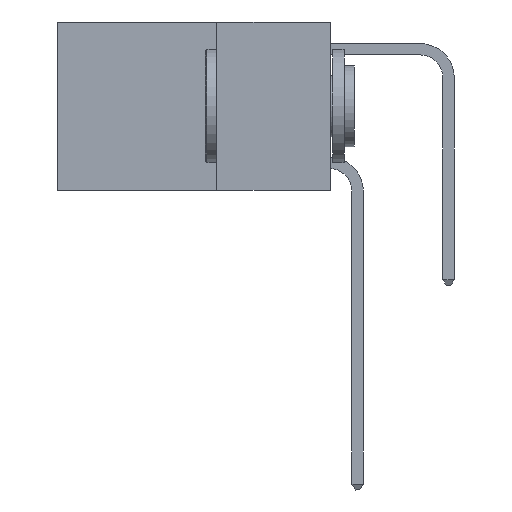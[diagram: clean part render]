
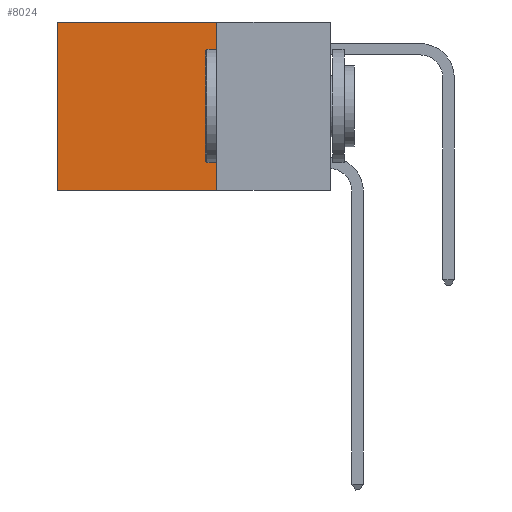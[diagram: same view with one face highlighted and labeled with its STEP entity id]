
A CAD part, left-side view. The second image highlights one B-rep face of the part: STEP entity #8024.
In plain terms, the highlighted planar face has unit normal (-1, 0, 0).
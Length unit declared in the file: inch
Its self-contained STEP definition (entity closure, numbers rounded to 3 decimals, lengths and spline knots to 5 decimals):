
#438 = DIRECTION ( 'NONE',  ( 0., 1., 0. ) ) ;
#1142 = VECTOR ( 'NONE', #12950, 39.37008 ) ;
#1522 = ORIENTED_EDGE ( 'NONE', *, *, #3613, .T. ) ;
#1818 = ORIENTED_EDGE ( 'NONE', *, *, #5618, .F. ) ;
#2028 = CARTESIAN_POINT ( 'NONE',  ( 0.2625, 0.6, 0. ) ) ;
#2216 = CARTESIAN_POINT ( 'NONE',  ( 0.2625, 0.25, 0. ) ) ;
#2420 = LINE ( 'NONE', #7058, #2683 ) ;
#2637 = VECTOR ( 'NONE', #438, 39.37008 ) ;
#2656 = CARTESIAN_POINT ( 'NONE',  ( 0.2625, 0.25, 0. ) ) ;
#2683 = VECTOR ( 'NONE', #15182, 39.37008 ) ;
#2760 = CARTESIAN_POINT ( 'NONE',  ( 0.2625, 0.6, 0. ) ) ;
#2827 = LINE ( 'NONE', #2760, #7575 ) ;
#3084 = VERTEX_POINT ( 'NONE', #2028 ) ;
#3613 = EDGE_CURVE ( 'NONE', #12579, #3084, #4598, .T. ) ;
#3783 = EDGE_CURVE ( 'NONE', #5805, #8089, #14579, .T. ) ;
#3784 = EDGE_CURVE ( 'NONE', #3084, #8089, #2827, .T. ) ;
#4338 = EDGE_LOOP ( 'NONE', ( #11737, #5523, #1818, #1522 ) ) ;
#4598 = LINE ( 'NONE', #2216, #1142 ) ;
#4959 = AXIS2_PLACEMENT_3D ( 'NONE', #7423, #13284, #6331 ) ;
#5523 = ORIENTED_EDGE ( 'NONE', *, *, #3783, .F. ) ;
#5618 = EDGE_CURVE ( 'NONE', #12579, #5805, #2420, .T. ) ;
#5805 = VERTEX_POINT ( 'NONE', #8611 ) ;
#6193 = FACE_OUTER_BOUND ( 'NONE', #4338, .T. ) ;
#6331 = DIRECTION ( 'NONE',  ( 0., 0., -1. ) ) ;
#7058 = CARTESIAN_POINT ( 'NONE',  ( 0.2625, 0.25, 0. ) ) ;
#7423 = CARTESIAN_POINT ( 'NONE',  ( 0.2625, 0.25, 0. ) ) ;
#7575 = VECTOR ( 'NONE', #11085, 39.37008 ) ;
#8024 = ADVANCED_FACE ( 'NONE', ( #6193 ), #8575, .F. ) ;
#8089 = VERTEX_POINT ( 'NONE', #9236 ) ;
#8575 = PLANE ( 'NONE',  #4959 ) ;
#8611 = CARTESIAN_POINT ( 'NONE',  ( 0.2625, 0.25, -0.37 ) ) ;
#9236 = CARTESIAN_POINT ( 'NONE',  ( 0.2625, 0.6, -0.37 ) ) ;
#10937 = CARTESIAN_POINT ( 'NONE',  ( 0.2625, 0.25, -0.37 ) ) ;
#11085 = DIRECTION ( 'NONE',  ( 0., 0., -1. ) ) ;
#11737 = ORIENTED_EDGE ( 'NONE', *, *, #3784, .T. ) ;
#12579 = VERTEX_POINT ( 'NONE', #2656 ) ;
#12950 = DIRECTION ( 'NONE',  ( 0., 1., 0. ) ) ;
#13284 = DIRECTION ( 'NONE',  ( 1., 0., 0. ) ) ;
#14579 = LINE ( 'NONE', #10937, #2637 ) ;
#15182 = DIRECTION ( 'NONE',  ( 0., 0., -1. ) ) ;
